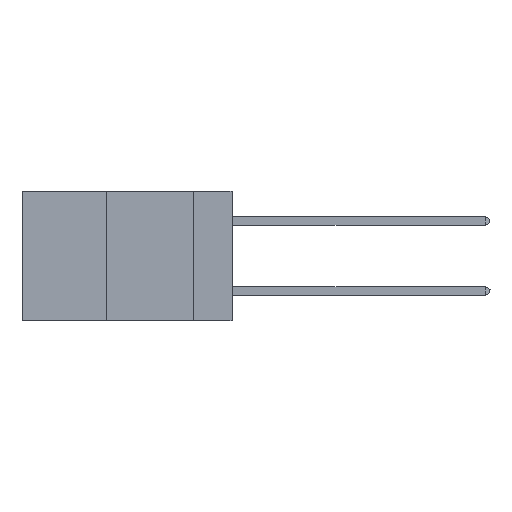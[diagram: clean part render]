
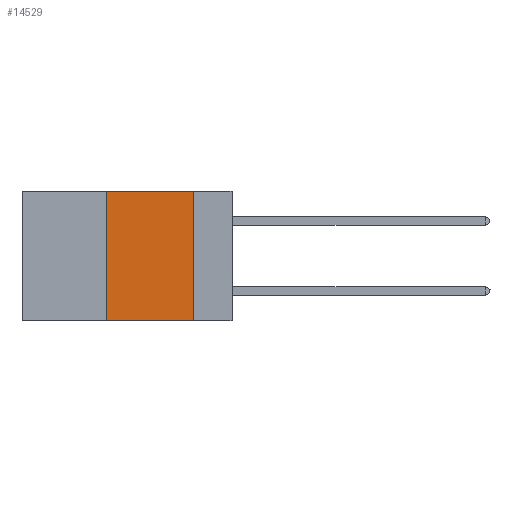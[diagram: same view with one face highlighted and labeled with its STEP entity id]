
A CAD part, left-side view. The second image highlights one B-rep face of the part: STEP entity #14529.
In plain terms, the highlighted planar face has unit normal (-1, 0, 0).
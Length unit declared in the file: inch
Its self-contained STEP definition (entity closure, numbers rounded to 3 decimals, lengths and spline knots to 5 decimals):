
#488 = LINE ( 'NONE', #15155, #5624 ) ;
#661 = DIRECTION ( 'NONE',  ( 0., 0., -1. ) ) ;
#1177 = ORIENTED_EDGE ( 'NONE', *, *, #24028, .F. ) ;
#2268 = PLANE ( 'NONE',  #10289 ) ;
#2705 = CARTESIAN_POINT ( 'NONE',  ( 0., 0.11, 0. ) ) ;
#4201 = DIRECTION ( 'NONE',  ( 0., -1., 0. ) ) ;
#4305 = FACE_OUTER_BOUND ( 'NONE', #25561, .T. ) ;
#5624 = VECTOR ( 'NONE', #14879, 39.37008 ) ;
#5798 = VERTEX_POINT ( 'NONE', #24383 ) ;
#6043 = ORIENTED_EDGE ( 'NONE', *, *, #23804, .T. ) ;
#6098 = VERTEX_POINT ( 'NONE', #15376 ) ;
#6254 = CARTESIAN_POINT ( 'NONE',  ( 0., 0.6, -0.37 ) ) ;
#6305 = VERTEX_POINT ( 'NONE', #6419 ) ;
#6419 = CARTESIAN_POINT ( 'NONE',  ( 0., 0.11, 0. ) ) ;
#6901 = DIRECTION ( 'NONE',  ( 0., 0., -1. ) ) ;
#7032 = DIRECTION ( 'NONE',  ( 1., 0., 0. ) ) ;
#7182 = ORIENTED_EDGE ( 'NONE', *, *, #18648, .F. ) ;
#8359 = VECTOR ( 'NONE', #661, 39.37008 ) ;
#10289 = AXIS2_PLACEMENT_3D ( 'NONE', #17467, #7032, #6901 ) ;
#10897 = LINE ( 'NONE', #16879, #17762 ) ;
#11036 = DIRECTION ( 'NONE',  ( 0., -1., 0. ) ) ;
#11990 = VERTEX_POINT ( 'NONE', #24317 ) ;
#13540 = LINE ( 'NONE', #2705, #8359 ) ;
#14529 = ADVANCED_FACE ( 'NONE', ( #4305 ), #2268, .F. ) ;
#14879 = DIRECTION ( 'NONE',  ( 0., 0., 1. ) ) ;
#15155 = CARTESIAN_POINT ( 'NONE',  ( 0., 0.36, 0. ) ) ;
#15376 = CARTESIAN_POINT ( 'NONE',  ( 0., 0.11, -0.37 ) ) ;
#16560 = VECTOR ( 'NONE', #4201, 39.37008 ) ;
#16879 = CARTESIAN_POINT ( 'NONE',  ( 0., 0.6, 0. ) ) ;
#17467 = CARTESIAN_POINT ( 'NONE',  ( 0., 0.6, 0. ) ) ;
#17762 = VECTOR ( 'NONE', #11036, 39.37008 ) ;
#18648 = EDGE_CURVE ( 'NONE', #11990, #5798, #488, .T. ) ;
#19133 = LINE ( 'NONE', #6254, #16560 ) ;
#19196 = EDGE_CURVE ( 'NONE', #5798, #6305, #10897, .T. ) ;
#19838 = ORIENTED_EDGE ( 'NONE', *, *, #19196, .F. ) ;
#23804 = EDGE_CURVE ( 'NONE', #11990, #6098, #19133, .T. ) ;
#24028 = EDGE_CURVE ( 'NONE', #6305, #6098, #13540, .T. ) ;
#24317 = CARTESIAN_POINT ( 'NONE',  ( 0., 0.36, -0.37 ) ) ;
#24383 = CARTESIAN_POINT ( 'NONE',  ( 0., 0.36, 0. ) ) ;
#25561 = EDGE_LOOP ( 'NONE', ( #1177, #19838, #7182, #6043 ) ) ;
